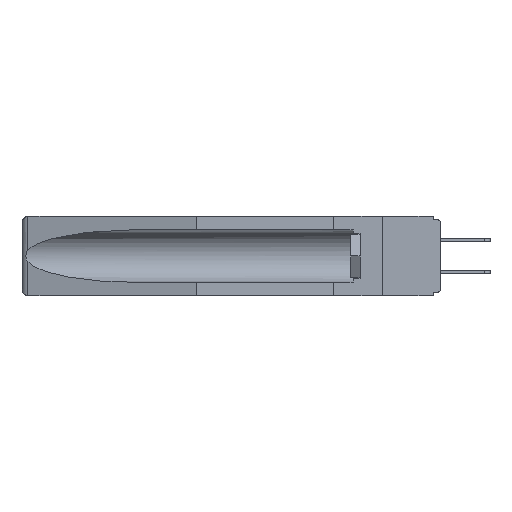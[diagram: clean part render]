
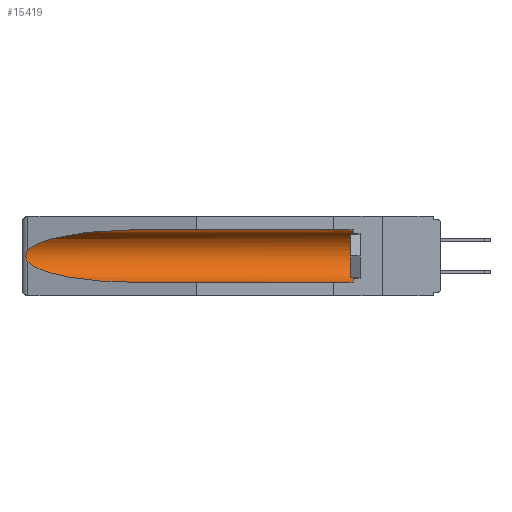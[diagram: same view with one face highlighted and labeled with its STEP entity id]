
A CAD part, left-side view. The second image highlights one B-rep face of the part: STEP entity #15419.
In plain terms, the highlighted cylindrical face has radius 2.857 mm (diameter 5.715 mm), a partial arc.
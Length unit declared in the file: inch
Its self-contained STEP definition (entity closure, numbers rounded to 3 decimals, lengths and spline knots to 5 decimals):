
#484 = EDGE_CURVE ( 'NONE', #10280, #9401, #9843, .T. ) ;
#500 = ORIENTED_EDGE ( 'NONE', *, *, #10683, .T. ) ;
#525 = AXIS2_PLACEMENT_3D ( 'NONE', #8277, #19147, #15883 ) ;
#1089 = VERTEX_POINT ( 'NONE', #16582 ) ;
#1585 = EDGE_CURVE ( 'NONE', #14257, #1089, #20422, .T. ) ;
#1818 = EDGE_CURVE ( 'NONE', #9401, #21840, #8350, .T. ) ;
#2281 = CARTESIAN_POINT ( 'NONE',  ( 0.26655, 1.53094, -0.18657 ) ) ;
#2422 = CARTESIAN_POINT ( 'NONE',  ( 0.155, -0.30754, -0.059 ) ) ;
#2552 = EDGE_CURVE ( 'NONE', #6489, #1089, #16336, .T. ) ;
#2925 = ORIENTED_EDGE ( 'NONE', *, *, #1585, .T. ) ;
#3665 = CARTESIAN_POINT ( 'NONE',  ( 0.26537, 1.52718, -0.14972 ) ) ;
#3673 = CARTESIAN_POINT ( 'NONE',  ( 0.26537, 1.52718, -0.19328 ) ) ;
#3688 = CARTESIAN_POINT ( 'NONE',  ( 0.155, 0.126, -0.1715 ) ) ;
#3972 = CARTESIAN_POINT ( 'NONE',  ( 0.2673, 1.53269, -0.17917 ) ) ;
#4345 = ORIENTED_EDGE ( 'NONE', *, *, #2552, .F. ) ;
#4392 = CARTESIAN_POINT ( 'NONE',  ( 0.26537, 1.52718, -0.14972 ) ) ;
#5066 = CYLINDRICAL_SURFACE ( 'NONE', #525, 0.1125 ) ;
#5594 = CARTESIAN_POINT ( 'NONE',  ( 0.26537, 1.52718, -0.14972 ) ) ;
#5882 = CARTESIAN_POINT ( 'NONE',  ( 0.155, 0.126, -0.284 ) ) ;
#6489 = VERTEX_POINT ( 'NONE', #5882 ) ;
#6622 = CARTESIAN_POINT ( 'NONE',  ( 0.155, -0.30754, -0.284 ) ) ;
#6852 = CARTESIAN_POINT ( 'NONE',  ( 0.155, 1.07973, -0.284 ) ) ;
#7299 = CARTESIAN_POINT ( 'NONE',  ( 0.2673, 1.5327, -0.16383 ) ) ;
#8277 = CARTESIAN_POINT ( 'NONE',  ( 0.155, -0.30754, -0.1715 ) ) ;
#8350 =( BOUNDED_CURVE ( )  B_SPLINE_CURVE ( 3, ( #20588, #13921, #13783, #3665 ),
 .UNSPECIFIED., .F., .F. ) 
 B_SPLINE_CURVE_WITH_KNOTS ( ( 4, 4 ),
 ( 4.71239, 6.08839 ),
 .UNSPECIFIED. ) 
 CURVE ( )  GEOMETRIC_REPRESENTATION_ITEM ( )  RATIONAL_B_SPLINE_CURVE ( ( 1., 0.848, 0.848, 1. ) ) 
 REPRESENTATION_ITEM ( '' )  );
#8444 = CIRCLE ( 'NONE', #10045, 0.1125 ) ;
#8760 = CARTESIAN_POINT ( 'NONE',  ( 0.26597, 1.52961, -0.15275 ) ) ;
#8984 = CARTESIAN_POINT ( 'NONE',  ( 0.2675, 1.53308, -0.16763 ) ) ;
#9129 = EDGE_CURVE ( 'NONE', #21840, #14257, #9968, .T. ) ;
#9401 = VERTEX_POINT ( 'NONE', #18868 ) ;
#9843 = LINE ( 'NONE', #2422, #16187 ) ;
#9968 = B_SPLINE_CURVE_WITH_KNOTS ( 'NONE', 3,
 ( #5594, #8760, #10684, #7299, #8984, #12390, #3972, #2281, #15503, #3673 ),
 .UNSPECIFIED., .F., .F.,
 ( 4, 2, 2, 2, 4 ),
 ( 0., 0.00029, 0.00058, 0.00087, 0.00117 ),
 .UNSPECIFIED. ) ;
#10045 = AXIS2_PLACEMENT_3D ( 'NONE', #3688, #13803, #14012 ) ;
#10280 = VERTEX_POINT ( 'NONE', #11769 ) ;
#10683 = EDGE_CURVE ( 'NONE', #6489, #10280, #8444, .T. ) ;
#10684 = CARTESIAN_POINT ( 'NONE',  ( 0.26654, 1.53092, -0.15636 ) ) ;
#10878 = FACE_OUTER_BOUND ( 'NONE', #12574, .T. ) ;
#10943 = ORIENTED_EDGE ( 'NONE', *, *, #9129, .T. ) ;
#11050 = DIRECTION ( 'NONE',  ( 0., 1., 0. ) ) ;
#11769 = CARTESIAN_POINT ( 'NONE',  ( 0.155, 0.126, -0.059 ) ) ;
#11817 = CARTESIAN_POINT ( 'NONE',  ( 0.26537, 1.52718, -0.19328 ) ) ;
#11877 = VECTOR ( 'NONE', #15106, 39.37008 ) ;
#11890 = CARTESIAN_POINT ( 'NONE',  ( 0.21114, 1.30732, -0.284 ) ) ;
#12390 = CARTESIAN_POINT ( 'NONE',  ( 0.2675, 1.53308, -0.17534 ) ) ;
#12574 = EDGE_LOOP ( 'NONE', ( #16940, #10943, #2925, #4345, #500, #18320 ) ) ;
#13783 = CARTESIAN_POINT ( 'NONE',  ( 0.25451, 1.48313, -0.09465 ) ) ;
#13803 = DIRECTION ( 'NONE',  ( 0., -1., 0. ) ) ;
#13921 = CARTESIAN_POINT ( 'NONE',  ( 0.21114, 1.30732, -0.059 ) ) ;
#14012 = DIRECTION ( 'NONE',  ( 0., 0., 1. ) ) ;
#14257 = VERTEX_POINT ( 'NONE', #19658 ) ;
#15106 = DIRECTION ( 'NONE',  ( 0., 1., 0. ) ) ;
#15419 = ADVANCED_FACE ( 'NONE', ( #10878 ), #5066, .F. ) ;
#15503 = CARTESIAN_POINT ( 'NONE',  ( 0.26597, 1.5296, -0.19026 ) ) ;
#15883 = DIRECTION ( 'NONE',  ( 0., 0., 1. ) ) ;
#16187 = VECTOR ( 'NONE', #11050, 39.37008 ) ;
#16336 = LINE ( 'NONE', #6622, #11877 ) ;
#16582 = CARTESIAN_POINT ( 'NONE',  ( 0.155, 1.07973, -0.284 ) ) ;
#16729 = CARTESIAN_POINT ( 'NONE',  ( 0.25451, 1.48313, -0.24835 ) ) ;
#16940 = ORIENTED_EDGE ( 'NONE', *, *, #1818, .T. ) ;
#18320 = ORIENTED_EDGE ( 'NONE', *, *, #484, .T. ) ;
#18868 = CARTESIAN_POINT ( 'NONE',  ( 0.155, 1.07973, -0.059 ) ) ;
#19147 = DIRECTION ( 'NONE',  ( 0., 1., 0. ) ) ;
#19658 = CARTESIAN_POINT ( 'NONE',  ( 0.26537, 1.52718, -0.19328 ) ) ;
#20422 =( BOUNDED_CURVE ( )  B_SPLINE_CURVE ( 3, ( #11817, #16729, #11890, #6852 ),
 .UNSPECIFIED., .F., .F. ) 
 B_SPLINE_CURVE_WITH_KNOTS ( ( 4, 4 ),
 ( 0.1948, 1.5708 ),
 .UNSPECIFIED. ) 
 CURVE ( )  GEOMETRIC_REPRESENTATION_ITEM ( )  RATIONAL_B_SPLINE_CURVE ( ( 1., 0.848, 0.848, 1. ) ) 
 REPRESENTATION_ITEM ( '' )  );
#20588 = CARTESIAN_POINT ( 'NONE',  ( 0.155, 1.07973, -0.059 ) ) ;
#21840 = VERTEX_POINT ( 'NONE', #4392 ) ;
